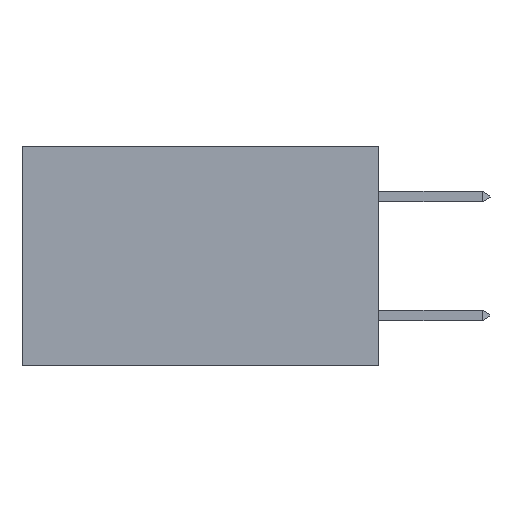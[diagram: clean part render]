
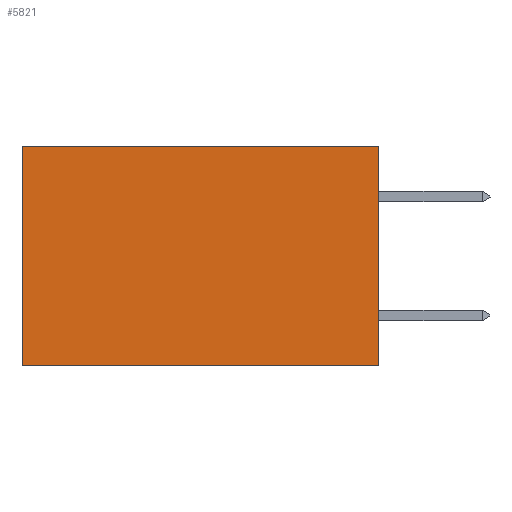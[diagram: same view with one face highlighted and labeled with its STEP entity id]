
A CAD part, left-side view. The second image highlights one B-rep face of the part: STEP entity #5821.
In plain terms, the highlighted planar face has unit normal (-1, 0, 0).
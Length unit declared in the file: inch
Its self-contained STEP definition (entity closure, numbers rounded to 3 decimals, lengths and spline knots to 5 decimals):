
#475 = CARTESIAN_POINT ( 'NONE',  ( 0.298, 0., -0.37 ) ) ;
#632 = CARTESIAN_POINT ( 'NONE',  ( 0.298, 0., 0. ) ) ;
#817 = CARTESIAN_POINT ( 'NONE',  ( 0.298, 0., -0.37 ) ) ;
#975 = CARTESIAN_POINT ( 'NONE',  ( 0.298, 0.6, 0. ) ) ;
#1027 = VECTOR ( 'NONE', #4811, 39.37008 ) ;
#1811 = ORIENTED_EDGE ( 'NONE', *, *, #6781, .F. ) ;
#2292 = DIRECTION ( 'NONE',  ( 0., 0., -1. ) ) ;
#2431 = LINE ( 'NONE', #817, #1027 ) ;
#2854 = CARTESIAN_POINT ( 'NONE',  ( 0.298, 0., 0. ) ) ;
#3152 = VERTEX_POINT ( 'NONE', #475 ) ;
#3468 = VECTOR ( 'NONE', #9440, 39.37008 ) ;
#3563 = CARTESIAN_POINT ( 'NONE',  ( 0.298, 0.6, 0. ) ) ;
#3828 = VECTOR ( 'NONE', #4169, 39.37008 ) ;
#3908 = VERTEX_POINT ( 'NONE', #3563 ) ;
#4090 = CARTESIAN_POINT ( 'NONE',  ( 0.298, 0., 0. ) ) ;
#4169 = DIRECTION ( 'NONE',  ( 0., 0., -1. ) ) ;
#4320 = LINE ( 'NONE', #975, #3828 ) ;
#4411 = EDGE_CURVE ( 'NONE', #10054, #3152, #6787, .T. ) ;
#4484 = LINE ( 'NONE', #2854, #3468 ) ;
#4811 = DIRECTION ( 'NONE',  ( 0., 1., 0. ) ) ;
#5565 = AXIS2_PLACEMENT_3D ( 'NONE', #632, #7152, #2292 ) ;
#5754 = VECTOR ( 'NONE', #7800, 39.37008 ) ;
#5757 = EDGE_CURVE ( 'NONE', #10054, #3908, #4484, .T. ) ;
#5821 = ADVANCED_FACE ( 'NONE', ( #6636 ), #8760, .F. ) ;
#6366 = EDGE_CURVE ( 'NONE', #3908, #6622, #4320, .T. ) ;
#6622 = VERTEX_POINT ( 'NONE', #7647 ) ;
#6636 = FACE_OUTER_BOUND ( 'NONE', #8876, .T. ) ;
#6781 = EDGE_CURVE ( 'NONE', #3152, #6622, #2431, .T. ) ;
#6787 = LINE ( 'NONE', #6993, #5754 ) ;
#6951 = ORIENTED_EDGE ( 'NONE', *, *, #6366, .T. ) ;
#6993 = CARTESIAN_POINT ( 'NONE',  ( 0.298, 0., 0. ) ) ;
#7152 = DIRECTION ( 'NONE',  ( 1., 0., 0. ) ) ;
#7647 = CARTESIAN_POINT ( 'NONE',  ( 0.298, 0.6, -0.37 ) ) ;
#7800 = DIRECTION ( 'NONE',  ( 0., 0., -1. ) ) ;
#8760 = PLANE ( 'NONE',  #5565 ) ;
#8876 = EDGE_LOOP ( 'NONE', ( #6951, #1811, #9693, #9098 ) ) ;
#9098 = ORIENTED_EDGE ( 'NONE', *, *, #5757, .T. ) ;
#9440 = DIRECTION ( 'NONE',  ( 0., 1., 0. ) ) ;
#9693 = ORIENTED_EDGE ( 'NONE', *, *, #4411, .F. ) ;
#10054 = VERTEX_POINT ( 'NONE', #4090 ) ;
